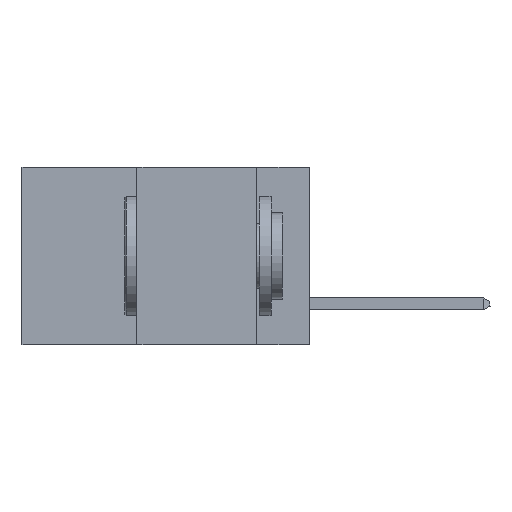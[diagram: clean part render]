
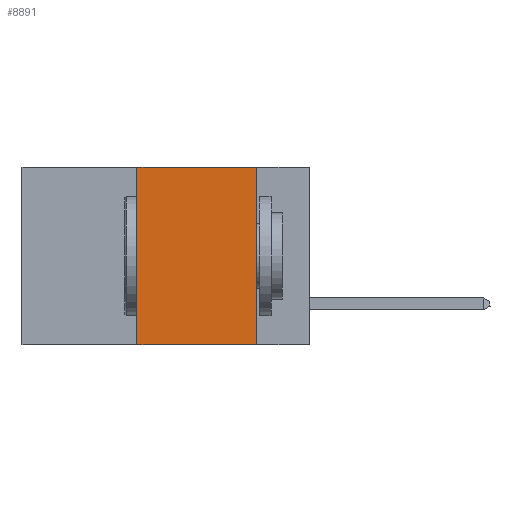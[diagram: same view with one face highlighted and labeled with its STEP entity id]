
A CAD part, left-side view. The second image highlights one B-rep face of the part: STEP entity #8891.
In plain terms, the highlighted planar face has unit normal (-1, 0, 0).
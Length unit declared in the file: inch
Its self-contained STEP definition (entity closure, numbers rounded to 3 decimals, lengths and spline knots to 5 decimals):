
#264 = ORIENTED_EDGE ( 'NONE', *, *, #8586, .F. ) ;
#2753 = FACE_OUTER_BOUND ( 'NONE', #21925, .T. ) ;
#3374 = ORIENTED_EDGE ( 'NONE', *, *, #32191, .T. ) ;
#4844 = LINE ( 'NONE', #28346, #31110 ) ;
#5841 = LINE ( 'NONE', #13436, #18299 ) ;
#7470 = VECTOR ( 'NONE', #16645, 39.37008 ) ;
#7735 = LINE ( 'NONE', #22955, #24659 ) ;
#8586 = EDGE_CURVE ( 'NONE', #26219, #35855, #5841, .T. ) ;
#8699 = PLANE ( 'NONE',  #34278 ) ;
#8891 = ADVANCED_FACE ( 'NONE', ( #2753 ), #8699, .F. ) ;
#9282 = LINE ( 'NONE', #32998, #7470 ) ;
#12328 = DIRECTION ( 'NONE',  ( 1., 0., 0. ) ) ;
#13436 = CARTESIAN_POINT ( 'NONE',  ( 0., 0.36, 0. ) ) ;
#13587 = EDGE_CURVE ( 'NONE', #15154, #35686, #7735, .T. ) ;
#15154 = VERTEX_POINT ( 'NONE', #28898 ) ;
#16645 = DIRECTION ( 'NONE',  ( 0., -1., 0. ) ) ;
#18299 = VECTOR ( 'NONE', #18699, 39.37008 ) ;
#18699 = DIRECTION ( 'NONE',  ( 0., 0., 1. ) ) ;
#21925 = EDGE_LOOP ( 'NONE', ( #34371, #31876, #264, #3374 ) ) ;
#22955 = CARTESIAN_POINT ( 'NONE',  ( 0., 0.11, 0. ) ) ;
#23190 = DIRECTION ( 'NONE',  ( 0., 0., -1. ) ) ;
#23580 = CARTESIAN_POINT ( 'NONE',  ( 0., 0.6, 0. ) ) ;
#23971 = DIRECTION ( 'NONE',  ( 0., 0., -1. ) ) ;
#24289 = CARTESIAN_POINT ( 'NONE',  ( 0., 0.36, 0. ) ) ;
#24659 = VECTOR ( 'NONE', #23190, 39.37008 ) ;
#25343 = DIRECTION ( 'NONE',  ( 0., -1., 0. ) ) ;
#26219 = VERTEX_POINT ( 'NONE', #27888 ) ;
#26865 = EDGE_CURVE ( 'NONE', #35855, #15154, #4844, .T. ) ;
#27888 = CARTESIAN_POINT ( 'NONE',  ( 0., 0.36, -0.37 ) ) ;
#28346 = CARTESIAN_POINT ( 'NONE',  ( 0., 0.6, 0. ) ) ;
#28898 = CARTESIAN_POINT ( 'NONE',  ( 0., 0.11, 0. ) ) ;
#31110 = VECTOR ( 'NONE', #25343, 39.37008 ) ;
#31876 = ORIENTED_EDGE ( 'NONE', *, *, #26865, .F. ) ;
#32191 = EDGE_CURVE ( 'NONE', #26219, #35686, #9282, .T. ) ;
#32690 = CARTESIAN_POINT ( 'NONE',  ( 0., 0.11, -0.37 ) ) ;
#32998 = CARTESIAN_POINT ( 'NONE',  ( 0., 0.6, -0.37 ) ) ;
#34278 = AXIS2_PLACEMENT_3D ( 'NONE', #23580, #12328, #23971 ) ;
#34371 = ORIENTED_EDGE ( 'NONE', *, *, #13587, .F. ) ;
#35686 = VERTEX_POINT ( 'NONE', #32690 ) ;
#35855 = VERTEX_POINT ( 'NONE', #24289 ) ;
